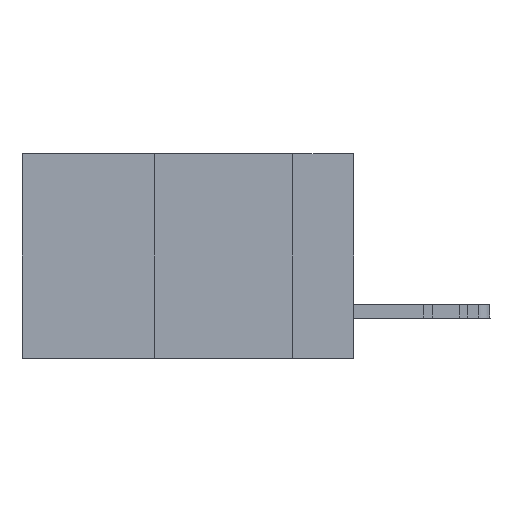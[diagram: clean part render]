
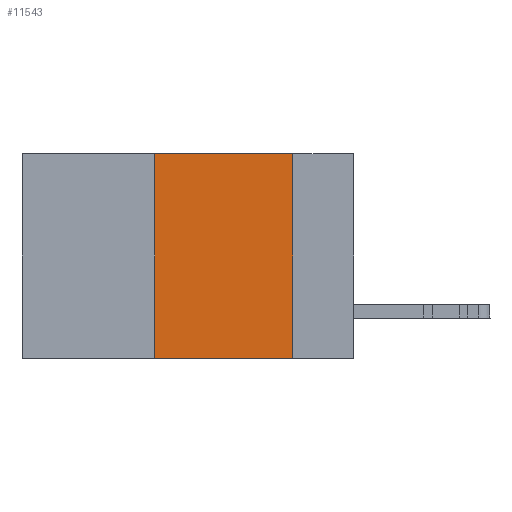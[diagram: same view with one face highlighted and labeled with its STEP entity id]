
A CAD part, left-side view. The second image highlights one B-rep face of the part: STEP entity #11543.
In plain terms, the highlighted planar face has unit normal (-1, 0, 0).
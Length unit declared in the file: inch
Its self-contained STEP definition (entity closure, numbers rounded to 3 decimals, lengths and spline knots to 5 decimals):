
#585 = EDGE_CURVE ( 'NONE', #38666, #2679, #38222, .T. ) ;
#1815 = EDGE_LOOP ( 'NONE', ( #34348, #23428, #25152, #3780 ) ) ;
#2617 = CARTESIAN_POINT ( 'NONE',  ( 0., 0.6, -0.37 ) ) ;
#2679 = VERTEX_POINT ( 'NONE', #10732 ) ;
#3780 = ORIENTED_EDGE ( 'NONE', *, *, #35251, .T. ) ;
#4455 = VERTEX_POINT ( 'NONE', #19568 ) ;
#6394 = VECTOR ( 'NONE', #11541, 39.37008 ) ;
#8136 = CARTESIAN_POINT ( 'NONE',  ( 0., 0.6, 0. ) ) ;
#10732 = CARTESIAN_POINT ( 'NONE',  ( 0., 0.36, 0. ) ) ;
#11541 = DIRECTION ( 'NONE',  ( 0., 0., -1. ) ) ;
#11543 = ADVANCED_FACE ( 'NONE', ( #29354 ), #25063, .F. ) ;
#11976 = CARTESIAN_POINT ( 'NONE',  ( 0., 0.11, 0. ) ) ;
#12148 = VERTEX_POINT ( 'NONE', #11976 ) ;
#12289 = DIRECTION ( 'NONE',  ( 0., 0., -1. ) ) ;
#12761 = VECTOR ( 'NONE', #41316, 39.37008 ) ;
#13992 = LINE ( 'NONE', #33730, #6394 ) ;
#16158 = LINE ( 'NONE', #2617, #40607 ) ;
#19568 = CARTESIAN_POINT ( 'NONE',  ( 0., 0.11, -0.37 ) ) ;
#22266 = CARTESIAN_POINT ( 'NONE',  ( 0., 0.36, 0. ) ) ;
#22602 = LINE ( 'NONE', #8136, #38505 ) ;
#23428 = ORIENTED_EDGE ( 'NONE', *, *, #26080, .F. ) ;
#24095 = CARTESIAN_POINT ( 'NONE',  ( 0., 0.36, -0.37 ) ) ;
#25063 = PLANE ( 'NONE',  #36353 ) ;
#25152 = ORIENTED_EDGE ( 'NONE', *, *, #585, .F. ) ;
#26080 = EDGE_CURVE ( 'NONE', #2679, #12148, #22602, .T. ) ;
#28226 = CARTESIAN_POINT ( 'NONE',  ( 0., 0.6, 0. ) ) ;
#29354 = FACE_OUTER_BOUND ( 'NONE', #1815, .T. ) ;
#31423 = DIRECTION ( 'NONE',  ( 1., 0., 0. ) ) ;
#33728 = DIRECTION ( 'NONE',  ( 0., -1., 0. ) ) ;
#33730 = CARTESIAN_POINT ( 'NONE',  ( 0., 0.11, 0. ) ) ;
#34348 = ORIENTED_EDGE ( 'NONE', *, *, #36969, .F. ) ;
#34765 = DIRECTION ( 'NONE',  ( 0., -1., 0. ) ) ;
#35251 = EDGE_CURVE ( 'NONE', #38666, #4455, #16158, .T. ) ;
#36353 = AXIS2_PLACEMENT_3D ( 'NONE', #28226, #31423, #12289 ) ;
#36969 = EDGE_CURVE ( 'NONE', #12148, #4455, #13992, .T. ) ;
#38222 = LINE ( 'NONE', #22266, #12761 ) ;
#38505 = VECTOR ( 'NONE', #33728, 39.37008 ) ;
#38666 = VERTEX_POINT ( 'NONE', #24095 ) ;
#40607 = VECTOR ( 'NONE', #34765, 39.37008 ) ;
#41316 = DIRECTION ( 'NONE',  ( 0., 0., 1. ) ) ;
